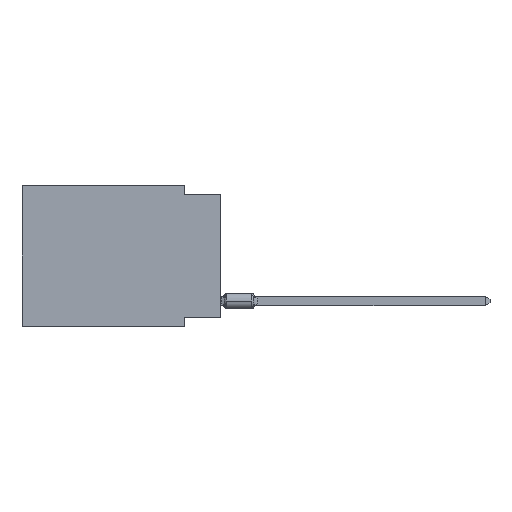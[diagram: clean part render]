
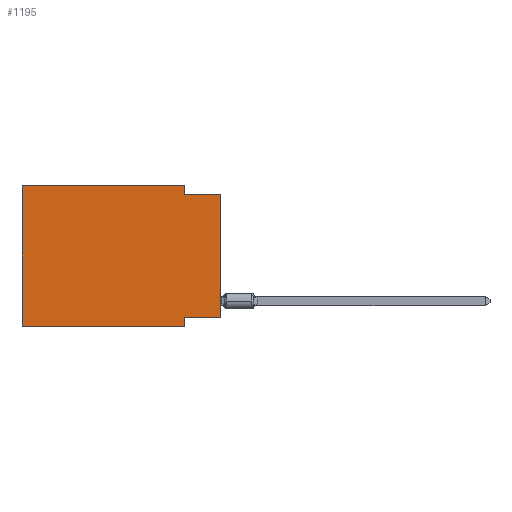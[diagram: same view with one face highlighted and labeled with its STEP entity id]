
A CAD part, left-side view. The second image highlights one B-rep face of the part: STEP entity #1195.
In plain terms, the highlighted planar face has unit normal (-1, 0, 0).
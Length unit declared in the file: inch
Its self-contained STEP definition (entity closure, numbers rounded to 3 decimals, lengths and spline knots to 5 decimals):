
#1195 = ADVANCED_FACE ( 'NONE', ( #6005 ), #6290, .F. ) ;
#1567 = VECTOR ( 'NONE', #44798, 39.37008 ) ;
#3364 = VERTEX_POINT ( 'NONE', #48065 ) ;
#5197 = CARTESIAN_POINT ( 'NONE',  ( 0., 0., -0.365 ) ) ;
#5814 = LINE ( 'NONE', #27795, #8501 ) ;
#6005 = FACE_OUTER_BOUND ( 'NONE', #8868, .T. ) ;
#6036 = CARTESIAN_POINT ( 'NONE',  ( 0., 0., -0.025 ) ) ;
#6290 = PLANE ( 'NONE',  #53356 ) ;
#6395 = ORIENTED_EDGE ( 'NONE', *, *, #13378, .T. ) ;
#7949 = LINE ( 'NONE', #17020, #44795 ) ;
#8501 = VECTOR ( 'NONE', #49790, 39.37008 ) ;
#8755 = LINE ( 'NONE', #5197, #19778 ) ;
#8868 = EDGE_LOOP ( 'NONE', ( #6395, #33968, #10338, #49299, #29101, #12077, #8969, #57512 ) ) ;
#8969 = ORIENTED_EDGE ( 'NONE', *, *, #15641, .F. ) ;
#9056 = LINE ( 'NONE', #26908, #1567 ) ;
#9884 = LINE ( 'NONE', #22797, #17672 ) ;
#10338 = ORIENTED_EDGE ( 'NONE', *, *, #23816, .F. ) ;
#12077 = ORIENTED_EDGE ( 'NONE', *, *, #21885, .T. ) ;
#13378 = EDGE_CURVE ( 'NONE', #19012, #39320, #9056, .T. ) ;
#14801 = CARTESIAN_POINT ( 'NONE',  ( 0., 0.55, 0. ) ) ;
#14905 = VERTEX_POINT ( 'NONE', #34200 ) ;
#15641 = EDGE_CURVE ( 'NONE', #27715, #3364, #56662, .T. ) ;
#16155 = EDGE_CURVE ( 'NONE', #19012, #27715, #8755, .T. ) ;
#16352 = VERTEX_POINT ( 'NONE', #51485 ) ;
#16474 = DIRECTION ( 'NONE',  ( 0., 0., -1. ) ) ;
#17020 = CARTESIAN_POINT ( 'NONE',  ( 0., 0.55, -0.39 ) ) ;
#17672 = VECTOR ( 'NONE', #50328, 39.37008 ) ;
#18938 = VECTOR ( 'NONE', #53700, 39.37008 ) ;
#19012 = VERTEX_POINT ( 'NONE', #53621 ) ;
#19778 = VECTOR ( 'NONE', #54164, 39.37008 ) ;
#19886 = EDGE_CURVE ( 'NONE', #50897, #40859, #36753, .T. ) ;
#21885 = EDGE_CURVE ( 'NONE', #16352, #3364, #7949, .T. ) ;
#22797 = CARTESIAN_POINT ( 'NONE',  ( 0., 0.1, 0. ) ) ;
#23816 = EDGE_CURVE ( 'NONE', #40859, #14905, #9884, .T. ) ;
#25581 = VECTOR ( 'NONE', #45845, 39.37008 ) ;
#26908 = CARTESIAN_POINT ( 'NONE',  ( 0., 0., 0. ) ) ;
#27715 = VERTEX_POINT ( 'NONE', #52941 ) ;
#27795 = CARTESIAN_POINT ( 'NONE',  ( 0., 0.55, 0. ) ) ;
#27949 = CARTESIAN_POINT ( 'NONE',  ( 0., 0.55, 0. ) ) ;
#29101 = ORIENTED_EDGE ( 'NONE', *, *, #53499, .F. ) ;
#30079 = CARTESIAN_POINT ( 'NONE',  ( 0., 0.55, 0. ) ) ;
#31114 = VECTOR ( 'NONE', #16474, 39.37008 ) ;
#33968 = ORIENTED_EDGE ( 'NONE', *, *, #55292, .F. ) ;
#34200 = CARTESIAN_POINT ( 'NONE',  ( 0., 0.1, -0.025 ) ) ;
#35790 = CARTESIAN_POINT ( 'NONE',  ( 0., 0., -0.025 ) ) ;
#36753 = LINE ( 'NONE', #27949, #25581 ) ;
#37943 = DIRECTION ( 'NONE',  ( 1., 0., 0. ) ) ;
#39320 = VERTEX_POINT ( 'NONE', #6036 ) ;
#40859 = VERTEX_POINT ( 'NONE', #57408 ) ;
#43144 = CARTESIAN_POINT ( 'NONE',  ( 0., 0.1, -0.39 ) ) ;
#44795 = VECTOR ( 'NONE', #48396, 39.37008 ) ;
#44798 = DIRECTION ( 'NONE',  ( 0., 0., 1. ) ) ;
#44881 = LINE ( 'NONE', #35790, #18938 ) ;
#45845 = DIRECTION ( 'NONE',  ( 0., -1., 0. ) ) ;
#48065 = CARTESIAN_POINT ( 'NONE',  ( 0., 0.1, -0.39 ) ) ;
#48396 = DIRECTION ( 'NONE',  ( 0., -1., 0. ) ) ;
#49299 = ORIENTED_EDGE ( 'NONE', *, *, #19886, .F. ) ;
#49790 = DIRECTION ( 'NONE',  ( 0., 0., 1. ) ) ;
#50328 = DIRECTION ( 'NONE',  ( 0., 0., -1. ) ) ;
#50560 = DIRECTION ( 'NONE',  ( 0., 0., -1. ) ) ;
#50897 = VERTEX_POINT ( 'NONE', #30079 ) ;
#51485 = CARTESIAN_POINT ( 'NONE',  ( 0., 0.55, -0.39 ) ) ;
#52941 = CARTESIAN_POINT ( 'NONE',  ( 0., 0.1, -0.365 ) ) ;
#53356 = AXIS2_PLACEMENT_3D ( 'NONE', #14801, #37943, #50560 ) ;
#53499 = EDGE_CURVE ( 'NONE', #16352, #50897, #5814, .T. ) ;
#53621 = CARTESIAN_POINT ( 'NONE',  ( 0., 0., -0.365 ) ) ;
#53700 = DIRECTION ( 'NONE',  ( 0., -1., 0. ) ) ;
#54164 = DIRECTION ( 'NONE',  ( 0., 1., 0. ) ) ;
#55292 = EDGE_CURVE ( 'NONE', #14905, #39320, #44881, .T. ) ;
#56662 = LINE ( 'NONE', #43144, #31114 ) ;
#57408 = CARTESIAN_POINT ( 'NONE',  ( 0., 0.1, 0. ) ) ;
#57512 = ORIENTED_EDGE ( 'NONE', *, *, #16155, .F. ) ;
